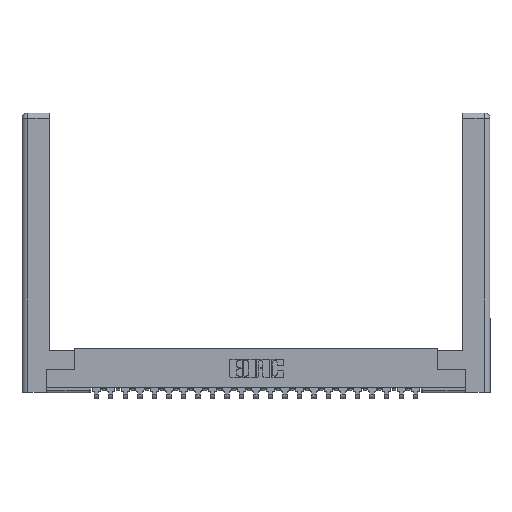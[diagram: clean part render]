
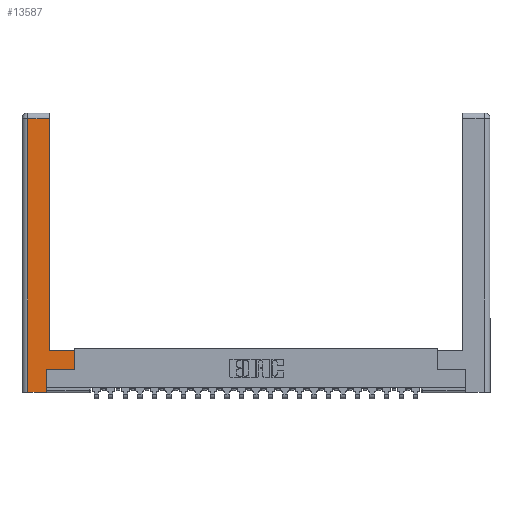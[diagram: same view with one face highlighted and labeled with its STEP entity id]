
A CAD part, top view. The second image highlights one B-rep face of the part: STEP entity #13587.
In plain terms, the highlighted planar face has unit normal (0, 0, 1).
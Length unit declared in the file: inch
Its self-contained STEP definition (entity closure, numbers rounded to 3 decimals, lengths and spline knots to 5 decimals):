
#478 = VECTOR ( 'NONE', #21936, 39.37008 ) ;
#519 = ORIENTED_EDGE ( 'NONE', *, *, #6721, .T. ) ;
#685 = DIRECTION ( 'NONE',  ( 0., 0., -1. ) ) ;
#983 = VERTEX_POINT ( 'NONE', #23904 ) ;
#996 = VERTEX_POINT ( 'NONE', #12752 ) ;
#1356 = VECTOR ( 'NONE', #20071, 39.37008 ) ;
#1682 = ORIENTED_EDGE ( 'NONE', *, *, #23899, .T. ) ;
#2377 = CARTESIAN_POINT ( 'NONE',  ( 0.565, 0.45, 0. ) ) ;
#2445 = DIRECTION ( 'NONE',  ( -1., 0., 0. ) ) ;
#2925 = CARTESIAN_POINT ( 'NONE',  ( 0.565, 0.45, 0. ) ) ;
#3090 = LINE ( 'NONE', #7222, #5139 ) ;
#4056 = ORIENTED_EDGE ( 'NONE', *, *, #9328, .T. ) ;
#4199 = VERTEX_POINT ( 'NONE', #19063 ) ;
#4466 = CARTESIAN_POINT ( 'NONE',  ( 0.265, 0., 0. ) ) ;
#4578 = PLANE ( 'NONE',  #19936 ) ;
#5139 = VECTOR ( 'NONE', #22032, 39.37008 ) ;
#5141 = EDGE_CURVE ( 'NONE', #10297, #16392, #9299, .T. ) ;
#5315 = CARTESIAN_POINT ( 'NONE',  ( 0.265, 0.245, 0. ) ) ;
#5599 = VERTEX_POINT ( 'NONE', #21086 ) ;
#6630 = CARTESIAN_POINT ( 'NONE',  ( 0.565, 0.245, 0. ) ) ;
#6721 = EDGE_CURVE ( 'NONE', #4199, #16791, #3090, .T. ) ;
#7222 = CARTESIAN_POINT ( 'NONE',  ( 0.0615, 2.94, 0. ) ) ;
#7680 = LINE ( 'NONE', #5315, #10731 ) ;
#8354 = DIRECTION ( 'NONE',  ( 1., 0., 0. ) ) ;
#8374 = EDGE_LOOP ( 'NONE', ( #21915, #519, #22366, #4056, #1682, #17920, #10568, #11438 ) ) ;
#9299 = LINE ( 'NONE', #17096, #14182 ) ;
#9328 = EDGE_CURVE ( 'NONE', #983, #5599, #16023, .T. ) ;
#10297 = VERTEX_POINT ( 'NONE', #2925 ) ;
#10529 = LINE ( 'NONE', #2377, #1356 ) ;
#10568 = ORIENTED_EDGE ( 'NONE', *, *, #18507, .T. ) ;
#10731 = VECTOR ( 'NONE', #12986, 39.37008 ) ;
#10922 = EDGE_CURVE ( 'NONE', #16392, #4199, #20693, .T. ) ;
#11172 = VERTEX_POINT ( 'NONE', #17432 ) ;
#11280 = CARTESIAN_POINT ( 'NONE',  ( 0.295, 3., 0. ) ) ;
#11438 = ORIENTED_EDGE ( 'NONE', *, *, #5141, .T. ) ;
#11881 = VECTOR ( 'NONE', #16832, 39.37008 ) ;
#12237 = CARTESIAN_POINT ( 'NONE',  ( 0., 0., 0. ) ) ;
#12650 = LINE ( 'NONE', #6630, #478 ) ;
#12752 = CARTESIAN_POINT ( 'NONE',  ( 0.265, 0.245, 0. ) ) ;
#12986 = DIRECTION ( 'NONE',  ( 0., 1., 0. ) ) ;
#13398 = CARTESIAN_POINT ( 'NONE',  ( 0.295, 0.45, 0. ) ) ;
#13587 = ADVANCED_FACE ( 'NONE', ( #21770 ), #4578, .F. ) ;
#13624 = DIRECTION ( 'NONE',  ( 0., -1., 0. ) ) ;
#14182 = VECTOR ( 'NONE', #16970, 39.37008 ) ;
#15869 = CARTESIAN_POINT ( 'NONE',  ( 0.0615, 0., 0. ) ) ;
#16023 = LINE ( 'NONE', #4466, #20073 ) ;
#16392 = VERTEX_POINT ( 'NONE', #13398 ) ;
#16791 = VERTEX_POINT ( 'NONE', #22642 ) ;
#16832 = DIRECTION ( 'NONE',  ( 0., 1., 0. ) ) ;
#16970 = DIRECTION ( 'NONE',  ( -1., 0., 0. ) ) ;
#17096 = CARTESIAN_POINT ( 'NONE',  ( 0.295, 0.45, 0. ) ) ;
#17432 = CARTESIAN_POINT ( 'NONE',  ( 0.565, 0.245, 0. ) ) ;
#17444 = EDGE_CURVE ( 'NONE', #996, #11172, #12650, .T. ) ;
#17920 = ORIENTED_EDGE ( 'NONE', *, *, #17444, .T. ) ;
#18507 = EDGE_CURVE ( 'NONE', #11172, #10297, #10529, .T. ) ;
#19063 = CARTESIAN_POINT ( 'NONE',  ( 0.295, 2.94, 0. ) ) ;
#19751 = LINE ( 'NONE', #15869, #21515 ) ;
#19936 = AXIS2_PLACEMENT_3D ( 'NONE', #12237, #685, #2445 ) ;
#20071 = DIRECTION ( 'NONE',  ( 0., 1., 0. ) ) ;
#20073 = VECTOR ( 'NONE', #8354, 39.37008 ) ;
#20693 = LINE ( 'NONE', #11280, #11881 ) ;
#21086 = CARTESIAN_POINT ( 'NONE',  ( 0.265, 0., 0. ) ) ;
#21515 = VECTOR ( 'NONE', #13624, 39.37008 ) ;
#21770 = FACE_OUTER_BOUND ( 'NONE', #8374, .T. ) ;
#21915 = ORIENTED_EDGE ( 'NONE', *, *, #10922, .T. ) ;
#21936 = DIRECTION ( 'NONE',  ( 1., 0., 0. ) ) ;
#22032 = DIRECTION ( 'NONE',  ( -1., 0., 0. ) ) ;
#22366 = ORIENTED_EDGE ( 'NONE', *, *, #23624, .T. ) ;
#22642 = CARTESIAN_POINT ( 'NONE',  ( 0.0615, 2.94, 0. ) ) ;
#23624 = EDGE_CURVE ( 'NONE', #16791, #983, #19751, .T. ) ;
#23899 = EDGE_CURVE ( 'NONE', #5599, #996, #7680, .T. ) ;
#23904 = CARTESIAN_POINT ( 'NONE',  ( 0.0615, 0., 0. ) ) ;
